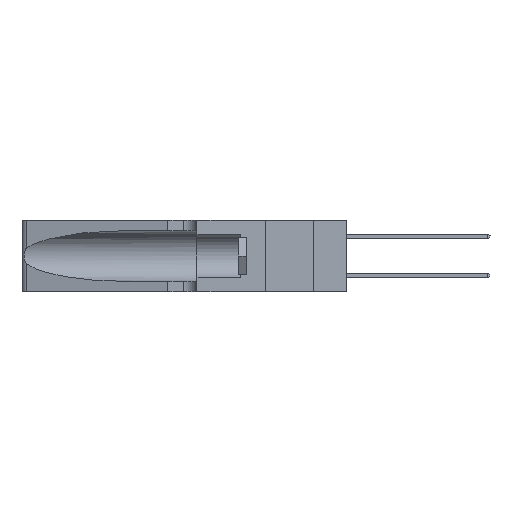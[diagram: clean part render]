
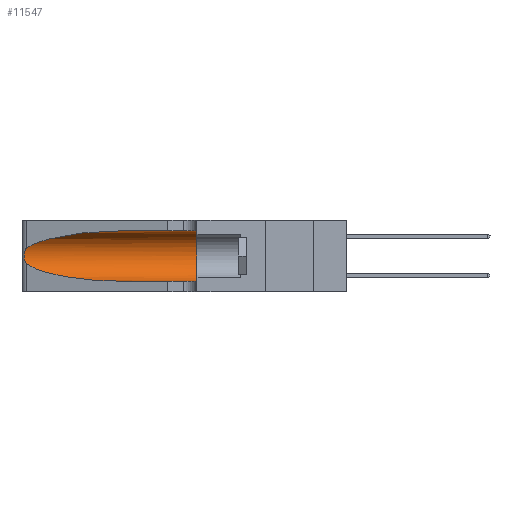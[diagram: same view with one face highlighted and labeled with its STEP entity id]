
A CAD part, left-side view. The second image highlights one B-rep face of the part: STEP entity #11547.
In plain terms, the highlighted cylindrical face has radius 3.308 mm (diameter 6.617 mm), a partial arc.
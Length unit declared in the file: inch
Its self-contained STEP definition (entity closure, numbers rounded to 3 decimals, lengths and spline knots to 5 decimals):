
#340 = CARTESIAN_POINT ( 'NONE',  ( 0.25487, 1.22718, 0.22369 ) ) ;
#412 = FACE_OUTER_BOUND ( 'NONE', #12932, .T. ) ;
#1852 = VERTEX_POINT ( 'NONE', #12139 ) ;
#2119 = CARTESIAN_POINT ( 'NONE',  ( 0.25789, 1.23486, 0.15765 ) ) ;
#2266 = AXIS2_PLACEMENT_3D ( 'NONE', #20248, #9180, #4681 ) ;
#2582 = EDGE_CURVE ( 'NONE', #8881, #6924, #17989, .T. ) ;
#2772 = DIRECTION ( 'NONE',  ( 0., -1., 0. ) ) ;
#3462 = EDGE_CURVE ( 'NONE', #21250, #1852, #18578, .T. ) ;
#4444 = CARTESIAN_POINT ( 'NONE',  ( 0.25555, 1.22993, 0.14849 ) ) ;
#4681 = DIRECTION ( 'NONE',  ( 0., 0., -1. ) ) ;
#6583 = CARTESIAN_POINT ( 'NONE',  ( 0.25555, 1.22994, 0.2215 ) ) ;
#6924 = VERTEX_POINT ( 'NONE', #26076 ) ;
#7092 = CIRCLE ( 'NONE', #24290, 0.13025 ) ;
#7322 = CARTESIAN_POINT ( 'NONE',  ( 0.1305, 1.61858, 0.05475 ) ) ;
#7553 = ORIENTED_EDGE ( 'NONE', *, *, #3462, .T. ) ;
#7975 = DIRECTION ( 'NONE',  ( 0., 1., 0. ) ) ;
#8201 = CARTESIAN_POINT ( 'NONE',  ( 0.1305, 0.72297, 0.05475 ) ) ;
#8717 = CARTESIAN_POINT ( 'NONE',  ( 0.1305, 0.35, 0.05475 ) ) ;
#8842 = CARTESIAN_POINT ( 'NONE',  ( 0.25787, 1.23484, 0.2124 ) ) ;
#8881 = VERTEX_POINT ( 'NONE', #22079 ) ;
#8941 = CYLINDRICAL_SURFACE ( 'NONE', #2266, 0.13025 ) ;
#9144 = ORIENTED_EDGE ( 'NONE', *, *, #2582, .F. ) ;
#9180 = DIRECTION ( 'NONE',  ( 0., -1., 0. ) ) ;
#9329 = CARTESIAN_POINT ( 'NONE',  ( 0.2373, 1.15595, 0.08982 ) ) ;
#9943 = CARTESIAN_POINT ( 'NONE',  ( 0.25487, 1.22718, 0.22369 ) ) ;
#10025 = ORIENTED_EDGE ( 'NONE', *, *, #12274, .T. ) ;
#11085 = ORIENTED_EDGE ( 'NONE', *, *, #28216, .T. ) ;
#11090 = CARTESIAN_POINT ( 'NONE',  ( 0.26018, 1.23835, 0.19895 ) ) ;
#11547 = ADVANCED_FACE ( 'NONE', ( #412 ), #8941, .F. ) ;
#11569 = CARTESIAN_POINT ( 'NONE',  ( 0.18966, 0.96281, 0.05475 ) ) ;
#11899 = LINE ( 'NONE', #7322, #17833 ) ;
#12139 = CARTESIAN_POINT ( 'NONE',  ( 0.25487, 1.22718, 0.14631 ) ) ;
#12274 = EDGE_CURVE ( 'NONE', #1852, #13338, #16471, .T. ) ;
#12485 = CARTESIAN_POINT ( 'NONE',  ( 0.1305, 1.61858, 0.31525 ) ) ;
#12932 = EDGE_LOOP ( 'NONE', ( #11085, #7553, #10025, #17475, #18320, #9144 ) ) ;
#13319 = CARTESIAN_POINT ( 'NONE',  ( 0.26075, 1.23896, 0.178 ) ) ;
#13338 = VERTEX_POINT ( 'NONE', #8201 ) ;
#13873 = CARTESIAN_POINT ( 'NONE',  ( 0.2373, 1.15595, 0.28018 ) ) ;
#13908 = EDGE_CURVE ( 'NONE', #6924, #22529, #7092, .T. ) ;
#14334 =( BOUNDED_CURVE ( )  B_SPLINE_CURVE ( 3, ( #16010, #26997, #13873, #340 ),
 .UNSPECIFIED., .F., .F. ) 
 B_SPLINE_CURVE_WITH_KNOTS ( ( 4, 4 ),
 ( 1.5708, 2.84003 ),
 .UNSPECIFIED. ) 
 CURVE ( )  GEOMETRIC_REPRESENTATION_ITEM ( )  RATIONAL_B_SPLINE_CURVE ( ( 1., 0.87, 0.87, 1. ) ) 
 REPRESENTATION_ITEM ( '' )  );
#15130 = EDGE_CURVE ( 'NONE', #13338, #22529, #11899, .T. ) ;
#15599 = CARTESIAN_POINT ( 'NONE',  ( 0.25856, 1.23593, 0.16098 ) ) ;
#16010 = CARTESIAN_POINT ( 'NONE',  ( 0.1305, 0.72297, 0.31525 ) ) ;
#16471 =( BOUNDED_CURVE ( )  B_SPLINE_CURVE ( 3, ( #22596, #9329, #11569, #26964 ),
 .UNSPECIFIED., .F., .F. ) 
 B_SPLINE_CURVE_WITH_KNOTS ( ( 4, 4 ),
 ( 3.44316, 4.71239 ),
 .UNSPECIFIED. ) 
 CURVE ( )  GEOMETRIC_REPRESENTATION_ITEM ( )  RATIONAL_B_SPLINE_CURVE ( ( 1., 0.87, 0.87, 1. ) ) 
 REPRESENTATION_ITEM ( '' )  );
#16608 = VECTOR ( 'NONE', #17078, 39.37008 ) ;
#17078 = DIRECTION ( 'NONE',  ( 0., -1., 0. ) ) ;
#17475 = ORIENTED_EDGE ( 'NONE', *, *, #15130, .T. ) ;
#17803 = CARTESIAN_POINT ( 'NONE',  ( 0.25639, 1.23186, 0.15144 ) ) ;
#17833 = VECTOR ( 'NONE', #2772, 39.37008 ) ;
#17989 = LINE ( 'NONE', #12485, #16608 ) ;
#18320 = ORIENTED_EDGE ( 'NONE', *, *, #13908, .F. ) ;
#18578 = B_SPLINE_CURVE_WITH_KNOTS ( 'NONE', 3,
 ( #19809, #6583, #22124, #8842, #24308, #11090, #26489, #13319, #28658, #15599, #2119, #17803, #4444, #20003 ),
 .UNSPECIFIED., .F., .F.,
 ( 4, 2, 2, 2, 2, 2, 4 ),
 ( 0., 0.00027, 0.00053, 0.00107, 0.0016, 0.00187, 0.00214 ),
 .UNSPECIFIED. ) ;
#19809 = CARTESIAN_POINT ( 'NONE',  ( 0.25487, 1.22718, 0.22369 ) ) ;
#20003 = CARTESIAN_POINT ( 'NONE',  ( 0.25487, 1.22718, 0.14631 ) ) ;
#20248 = CARTESIAN_POINT ( 'NONE',  ( 0.1305, 1.61858, 0.185 ) ) ;
#21250 = VERTEX_POINT ( 'NONE', #9943 ) ;
#21266 = CARTESIAN_POINT ( 'NONE',  ( 0.1305, 0.35, 0.185 ) ) ;
#22079 = CARTESIAN_POINT ( 'NONE',  ( 0.1305, 0.72297, 0.31525 ) ) ;
#22124 = CARTESIAN_POINT ( 'NONE',  ( 0.25639, 1.23184, 0.21858 ) ) ;
#22529 = VERTEX_POINT ( 'NONE', #8717 ) ;
#22596 = CARTESIAN_POINT ( 'NONE',  ( 0.25487, 1.22718, 0.14631 ) ) ;
#23450 = DIRECTION ( 'NONE',  ( 0., 0., 1. ) ) ;
#24290 = AXIS2_PLACEMENT_3D ( 'NONE', #21266, #7975, #23450 ) ;
#24308 = CARTESIAN_POINT ( 'NONE',  ( 0.25854, 1.2359, 0.20912 ) ) ;
#26076 = CARTESIAN_POINT ( 'NONE',  ( 0.1305, 0.35, 0.31525 ) ) ;
#26489 = CARTESIAN_POINT ( 'NONE',  ( 0.26075, 1.23896, 0.19203 ) ) ;
#26964 = CARTESIAN_POINT ( 'NONE',  ( 0.1305, 0.72297, 0.05475 ) ) ;
#26997 = CARTESIAN_POINT ( 'NONE',  ( 0.18966, 0.96281, 0.31525 ) ) ;
#28216 = EDGE_CURVE ( 'NONE', #8881, #21250, #14334, .T. ) ;
#28658 = CARTESIAN_POINT ( 'NONE',  ( 0.26017, 1.23833, 0.17102 ) ) ;
